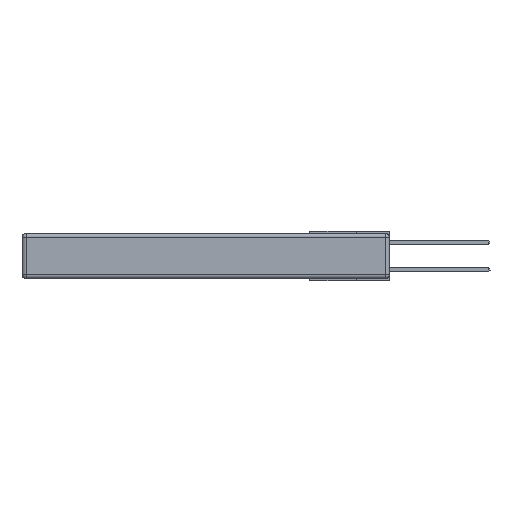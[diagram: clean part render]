
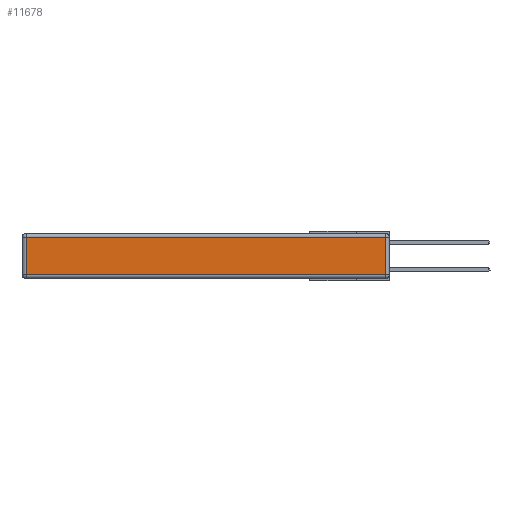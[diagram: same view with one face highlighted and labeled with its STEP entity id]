
A CAD part, left-side view. The second image highlights one B-rep face of the part: STEP entity #11678.
In plain terms, the highlighted planar face has unit normal (-1, 0, 0).
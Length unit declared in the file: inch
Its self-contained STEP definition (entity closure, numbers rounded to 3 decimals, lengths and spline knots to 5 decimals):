
#889 = VECTOR ( 'NONE', #5288, 39.37008 ) ;
#1891 = DIRECTION ( 'NONE',  ( 0., -1., 0. ) ) ;
#3313 = DIRECTION ( 'NONE',  ( 0., 1., 0. ) ) ;
#3546 = CARTESIAN_POINT ( 'NONE',  ( 0., 0.03, -0.343 ) ) ;
#4203 = VERTEX_POINT ( 'NONE', #21130 ) ;
#4726 = LINE ( 'NONE', #3546, #889 ) ;
#4883 = DIRECTION ( 'NONE',  ( 0., 0., -1. ) ) ;
#5288 = DIRECTION ( 'NONE',  ( 0., 0., 1. ) ) ;
#5298 = VECTOR ( 'NONE', #3313, 39.37008 ) ;
#5376 = CARTESIAN_POINT ( 'NONE',  ( 0., 2.72, -0.313 ) ) ;
#5621 = EDGE_CURVE ( 'NONE', #7377, #9855, #9523, .T. ) ;
#7331 = EDGE_CURVE ( 'NONE', #12971, #4203, #11029, .T. ) ;
#7377 = VERTEX_POINT ( 'NONE', #5376 ) ;
#7891 = CARTESIAN_POINT ( 'NONE',  ( 0., 0., -0.313 ) ) ;
#7947 = EDGE_CURVE ( 'NONE', #4203, #7377, #20582, .T. ) ;
#8559 = CARTESIAN_POINT ( 'NONE',  ( 0., 0., -0.343 ) ) ;
#9523 = LINE ( 'NONE', #7891, #20089 ) ;
#9758 = ORIENTED_EDGE ( 'NONE', *, *, #7331, .T. ) ;
#9855 = VERTEX_POINT ( 'NONE', #10467 ) ;
#10070 = VECTOR ( 'NONE', #4883, 39.37008 ) ;
#10467 = CARTESIAN_POINT ( 'NONE',  ( 0., 0.03, -0.313 ) ) ;
#11029 = LINE ( 'NONE', #20672, #5298 ) ;
#11678 = ADVANCED_FACE ( 'NONE', ( #19051 ), #16215, .T. ) ;
#12971 = VERTEX_POINT ( 'NONE', #21568 ) ;
#16215 = PLANE ( 'NONE',  #20164 ) ;
#17482 = EDGE_CURVE ( 'NONE', #9855, #12971, #4726, .T. ) ;
#18246 = CARTESIAN_POINT ( 'NONE',  ( 0., 2.72, -0.343 ) ) ;
#18350 = EDGE_LOOP ( 'NONE', ( #23715, #23636, #9758, #20428 ) ) ;
#19051 = FACE_OUTER_BOUND ( 'NONE', #18350, .T. ) ;
#20089 = VECTOR ( 'NONE', #1891, 39.37008 ) ;
#20164 = AXIS2_PLACEMENT_3D ( 'NONE', #8559, #24040, #21926 ) ;
#20428 = ORIENTED_EDGE ( 'NONE', *, *, #7947, .T. ) ;
#20582 = LINE ( 'NONE', #18246, #10070 ) ;
#20672 = CARTESIAN_POINT ( 'NONE',  ( 0., 2.75, -0.03 ) ) ;
#21130 = CARTESIAN_POINT ( 'NONE',  ( 0., 2.72, -0.03 ) ) ;
#21568 = CARTESIAN_POINT ( 'NONE',  ( 0., 0.03, -0.03 ) ) ;
#21926 = DIRECTION ( 'NONE',  ( 0., 0., 1. ) ) ;
#23636 = ORIENTED_EDGE ( 'NONE', *, *, #17482, .T. ) ;
#23715 = ORIENTED_EDGE ( 'NONE', *, *, #5621, .T. ) ;
#24040 = DIRECTION ( 'NONE',  ( -1., 0., 0. ) ) ;
